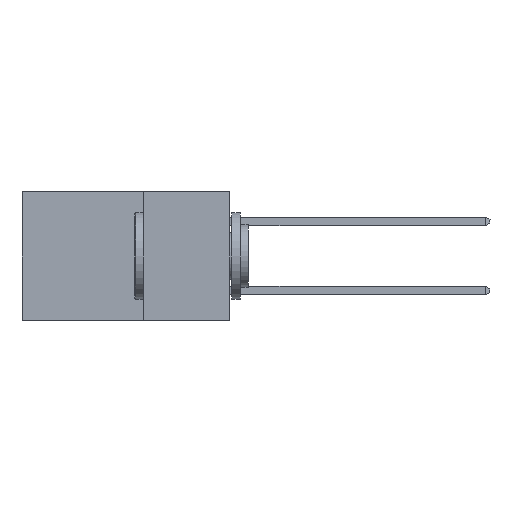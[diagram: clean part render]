
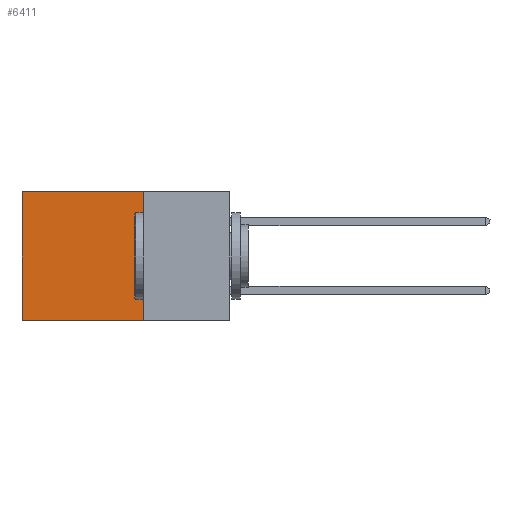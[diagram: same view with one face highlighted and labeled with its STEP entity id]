
A CAD part, left-side view. The second image highlights one B-rep face of the part: STEP entity #6411.
In plain terms, the highlighted planar face has unit normal (-1, 0, 0).
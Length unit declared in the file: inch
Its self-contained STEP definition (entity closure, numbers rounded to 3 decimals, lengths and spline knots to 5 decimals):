
#154 = DIRECTION ( 'NONE',  ( 0., 1., 0. ) ) ;
#227 = CARTESIAN_POINT ( 'NONE',  ( 0.2615, 0.25, -0.37 ) ) ;
#973 = DIRECTION ( 'NONE',  ( 1., 0., 0. ) ) ;
#1178 = CARTESIAN_POINT ( 'NONE',  ( 0.2615, 0.6, -0.37 ) ) ;
#1229 = DIRECTION ( 'NONE',  ( 0., 0., -1. ) ) ;
#1486 = CARTESIAN_POINT ( 'NONE',  ( 0.2615, 0.25, 0. ) ) ;
#1821 = LINE ( 'NONE', #2579, #3642 ) ;
#2078 = EDGE_LOOP ( 'NONE', ( #7666, #7944, #7180, #4070 ) ) ;
#2199 = CARTESIAN_POINT ( 'NONE',  ( 0.2615, 0.25, -0.37 ) ) ;
#2288 = AXIS2_PLACEMENT_3D ( 'NONE', #227, #973, #6747 ) ;
#2579 = CARTESIAN_POINT ( 'NONE',  ( 0.2615, 0.25, -0.37 ) ) ;
#2969 = EDGE_CURVE ( 'NONE', #10053, #3347, #4960, .T. ) ;
#3007 = DIRECTION ( 'NONE',  ( 0., 1., 0. ) ) ;
#3040 = VERTEX_POINT ( 'NONE', #4636 ) ;
#3347 = VERTEX_POINT ( 'NONE', #7470 ) ;
#3415 = CARTESIAN_POINT ( 'NONE',  ( 0.2615, 0.25, 0. ) ) ;
#3490 = FACE_OUTER_BOUND ( 'NONE', #2078, .T. ) ;
#3642 = VECTOR ( 'NONE', #8253, 39.37008 ) ;
#4017 = LINE ( 'NONE', #2199, #7923 ) ;
#4070 = ORIENTED_EDGE ( 'NONE', *, *, #2969, .T. ) ;
#4449 = EDGE_CURVE ( 'NONE', #3347, #3040, #10151, .T. ) ;
#4595 = CARTESIAN_POINT ( 'NONE',  ( 0.2615, 0.25, -0.37 ) ) ;
#4636 = CARTESIAN_POINT ( 'NONE',  ( 0.2615, 0.6, -0.37 ) ) ;
#4657 = VECTOR ( 'NONE', #1229, 39.37008 ) ;
#4960 = LINE ( 'NONE', #3415, #4961 ) ;
#4961 = VECTOR ( 'NONE', #154, 39.37008 ) ;
#5609 = EDGE_CURVE ( 'NONE', #8294, #3040, #4017, .T. ) ;
#6349 = EDGE_CURVE ( 'NONE', #10053, #8294, #1821, .T. ) ;
#6411 = ADVANCED_FACE ( 'NONE', ( #3490 ), #8304, .F. ) ;
#6747 = DIRECTION ( 'NONE',  ( 0., 0., -1. ) ) ;
#7180 = ORIENTED_EDGE ( 'NONE', *, *, #6349, .F. ) ;
#7470 = CARTESIAN_POINT ( 'NONE',  ( 0.2615, 0.6, 0. ) ) ;
#7666 = ORIENTED_EDGE ( 'NONE', *, *, #4449, .T. ) ;
#7923 = VECTOR ( 'NONE', #3007, 39.37008 ) ;
#7944 = ORIENTED_EDGE ( 'NONE', *, *, #5609, .F. ) ;
#8253 = DIRECTION ( 'NONE',  ( 0., 0., -1. ) ) ;
#8294 = VERTEX_POINT ( 'NONE', #4595 ) ;
#8304 = PLANE ( 'NONE',  #2288 ) ;
#10053 = VERTEX_POINT ( 'NONE', #1486 ) ;
#10151 = LINE ( 'NONE', #1178, #4657 ) ;
